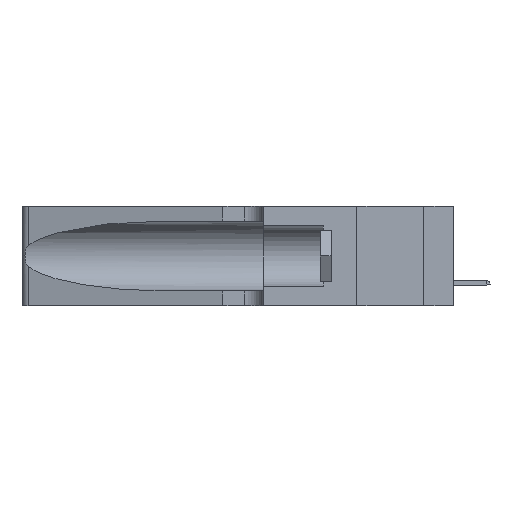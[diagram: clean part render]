
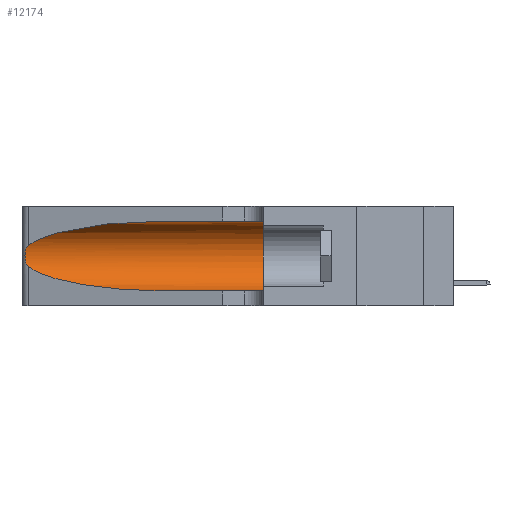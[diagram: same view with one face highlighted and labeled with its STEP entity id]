
A CAD part, left-side view. The second image highlights one B-rep face of the part: STEP entity #12174.
In plain terms, the highlighted cylindrical face has radius 3.308 mm (diameter 6.617 mm), a partial arc.
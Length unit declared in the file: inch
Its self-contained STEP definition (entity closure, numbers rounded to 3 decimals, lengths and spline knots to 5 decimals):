
#591 = CARTESIAN_POINT ( 'NONE',  ( 0.25789, 1.23486, 0.15765 ) ) ;
#1418 = EDGE_CURVE ( 'NONE', #18678, #30927, #24398, .T. ) ;
#3069 = CARTESIAN_POINT ( 'NONE',  ( 0.25487, 1.22718, 0.22369 ) ) ;
#4185 = CARTESIAN_POINT ( 'NONE',  ( 0.2373, 1.15595, 0.08982 ) ) ;
#4538 = CARTESIAN_POINT ( 'NONE',  ( 0.25854, 1.2359, 0.20912 ) ) ;
#4629 = VERTEX_POINT ( 'NONE', #37437 ) ;
#4692 = EDGE_CURVE ( 'NONE', #4629, #18678, #28216, .T. ) ;
#5377 = ORIENTED_EDGE ( 'NONE', *, *, #23769, .F. ) ;
#5863 =( BOUNDED_CURVE ( )  B_SPLINE_CURVE ( 3, ( #39801, #39375, #20364, #3069 ),
 .UNSPECIFIED., .F., .T. ) 
 B_SPLINE_CURVE_WITH_KNOTS ( ( 4, 4 ),
 ( 1.5708, 2.84003 ),
 .UNSPECIFIED. ) 
 CURVE ( )  GEOMETRIC_REPRESENTATION_ITEM ( )  RATIONAL_B_SPLINE_CURVE ( ( 1., 0.87, 0.87, 1. ) ) 
 REPRESENTATION_ITEM ( '' )  );
#6408 = CARTESIAN_POINT ( 'NONE',  ( 0.1305, 1.61858, 0.31525 ) ) ;
#7145 = ORIENTED_EDGE ( 'NONE', *, *, #15708, .F. ) ;
#7391 = CARTESIAN_POINT ( 'NONE',  ( 0.25555, 1.22994, 0.2215 ) ) ;
#7828 = CARTESIAN_POINT ( 'NONE',  ( 0.25639, 1.23184, 0.21858 ) ) ;
#7927 = CIRCLE ( 'NONE', #35157, 0.13025 ) ;
#7989 = CARTESIAN_POINT ( 'NONE',  ( 0.1305, 1.61858, 0.05475 ) ) ;
#8183 = VECTOR ( 'NONE', #10407, 39.37008 ) ;
#9133 = ORIENTED_EDGE ( 'NONE', *, *, #1418, .T. ) ;
#9334 = VERTEX_POINT ( 'NONE', #29270 ) ;
#10407 = DIRECTION ( 'NONE',  ( 0., -1., 0. ) ) ;
#10449 = CARTESIAN_POINT ( 'NONE',  ( 0.25856, 1.23593, 0.16098 ) ) ;
#10877 = CARTESIAN_POINT ( 'NONE',  ( 0.26075, 1.23896, 0.178 ) ) ;
#11068 = DIRECTION ( 'NONE',  ( 0., 0., -1. ) ) ;
#11296 = DIRECTION ( 'NONE',  ( 0., -1., 0. ) ) ;
#11319 = CARTESIAN_POINT ( 'NONE',  ( 0.26017, 1.23833, 0.17102 ) ) ;
#12071 = DIRECTION ( 'NONE',  ( 0., 1., 0. ) ) ;
#12174 = ADVANCED_FACE ( 'NONE', ( #21153 ), #28142, .F. ) ;
#12304 = DIRECTION ( 'NONE',  ( 0., -1., 0. ) ) ;
#12371 = ORIENTED_EDGE ( 'NONE', *, *, #19377, .T. ) ;
#13672 = CARTESIAN_POINT ( 'NONE',  ( 0.1305, 0.35, 0.05475 ) ) ;
#13895 = CARTESIAN_POINT ( 'NONE',  ( 0.1305, 0.72297, 0.31525 ) ) ;
#14239 = CARTESIAN_POINT ( 'NONE',  ( 0.18966, 0.96281, 0.05475 ) ) ;
#15708 = EDGE_CURVE ( 'NONE', #32327, #9334, #28939, .T. ) ;
#17890 = CARTESIAN_POINT ( 'NONE',  ( 0.26075, 1.23896, 0.19203 ) ) ;
#18434 = DIRECTION ( 'NONE',  ( 0., 0., 1. ) ) ;
#18678 = VERTEX_POINT ( 'NONE', #27614 ) ;
#19377 = EDGE_CURVE ( 'NONE', #24435, #4629, #27220, .T. ) ;
#20364 = CARTESIAN_POINT ( 'NONE',  ( 0.2373, 1.15595, 0.28018 ) ) ;
#20536 = CARTESIAN_POINT ( 'NONE',  ( 0.25555, 1.22993, 0.14849 ) ) ;
#20750 = CARTESIAN_POINT ( 'NONE',  ( 0.25487, 1.22718, 0.14631 ) ) ;
#21153 = FACE_OUTER_BOUND ( 'NONE', #32505, .T. ) ;
#21491 = VECTOR ( 'NONE', #12304, 39.37008 ) ;
#22792 = AXIS2_PLACEMENT_3D ( 'NONE', #41253, #11296, #11068 ) ;
#23769 = EDGE_CURVE ( 'NONE', #9334, #30927, #7927, .T. ) ;
#24398 = LINE ( 'NONE', #7989, #8183 ) ;
#24435 = VERTEX_POINT ( 'NONE', #35427 ) ;
#24451 = CARTESIAN_POINT ( 'NONE',  ( 0.25787, 1.23484, 0.2124 ) ) ;
#27220 = B_SPLINE_CURVE_WITH_KNOTS ( 'NONE', 3,
 ( #40841, #7391, #7828, #24451, #4538, #37361, #17890, #10877, #11319, #10449, #591, #34295, #20536, #20750 ),
 .UNSPECIFIED., .F., .F.,
 ( 4, 2, 2, 2, 2, 2, 4 ),
 ( 0., 0.00027, 0.00053, 0.00107, 0.0016, 0.00187, 0.00214 ),
 .UNSPECIFIED. ) ;
#27591 = CARTESIAN_POINT ( 'NONE',  ( 0.1305, 0.72297, 0.05475 ) ) ;
#27614 = CARTESIAN_POINT ( 'NONE',  ( 0.1305, 0.72297, 0.05475 ) ) ;
#28142 = CYLINDRICAL_SURFACE ( 'NONE', #22792, 0.13025 ) ;
#28216 =( BOUNDED_CURVE ( )  B_SPLINE_CURVE ( 3, ( #34155, #4185, #14239, #27591 ),
 .UNSPECIFIED., .F., .T. ) 
 B_SPLINE_CURVE_WITH_KNOTS ( ( 4, 4 ),
 ( 3.44316, 4.71239 ),
 .UNSPECIFIED. ) 
 CURVE ( )  GEOMETRIC_REPRESENTATION_ITEM ( )  RATIONAL_B_SPLINE_CURVE ( ( 1., 0.87, 0.87, 1. ) ) 
 REPRESENTATION_ITEM ( '' )  );
#28219 = ORIENTED_EDGE ( 'NONE', *, *, #33877, .T. ) ;
#28939 = LINE ( 'NONE', #6408, #21491 ) ;
#29270 = CARTESIAN_POINT ( 'NONE',  ( 0.1305, 0.35, 0.31525 ) ) ;
#30927 = VERTEX_POINT ( 'NONE', #13672 ) ;
#32327 = VERTEX_POINT ( 'NONE', #13895 ) ;
#32505 = EDGE_LOOP ( 'NONE', ( #28219, #12371, #41604, #9133, #5377, #7145 ) ) ;
#33877 = EDGE_CURVE ( 'NONE', #32327, #24435, #5863, .T. ) ;
#34155 = CARTESIAN_POINT ( 'NONE',  ( 0.25487, 1.22718, 0.14631 ) ) ;
#34295 = CARTESIAN_POINT ( 'NONE',  ( 0.25639, 1.23186, 0.15144 ) ) ;
#35157 = AXIS2_PLACEMENT_3D ( 'NONE', #42041, #12071, #18434 ) ;
#35427 = CARTESIAN_POINT ( 'NONE',  ( 0.25487, 1.22718, 0.22369 ) ) ;
#37361 = CARTESIAN_POINT ( 'NONE',  ( 0.26018, 1.23835, 0.19895 ) ) ;
#37437 = CARTESIAN_POINT ( 'NONE',  ( 0.25487, 1.22718, 0.14631 ) ) ;
#39375 = CARTESIAN_POINT ( 'NONE',  ( 0.18966, 0.96281, 0.31525 ) ) ;
#39801 = CARTESIAN_POINT ( 'NONE',  ( 0.1305, 0.72297, 0.31525 ) ) ;
#40841 = CARTESIAN_POINT ( 'NONE',  ( 0.25487, 1.22718, 0.22369 ) ) ;
#41253 = CARTESIAN_POINT ( 'NONE',  ( 0.1305, 1.61858, 0.185 ) ) ;
#41604 = ORIENTED_EDGE ( 'NONE', *, *, #4692, .T. ) ;
#42041 = CARTESIAN_POINT ( 'NONE',  ( 0.1305, 0.35, 0.185 ) ) ;
